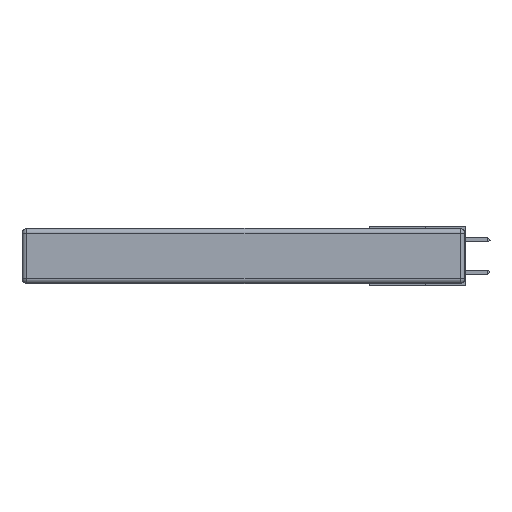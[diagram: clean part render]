
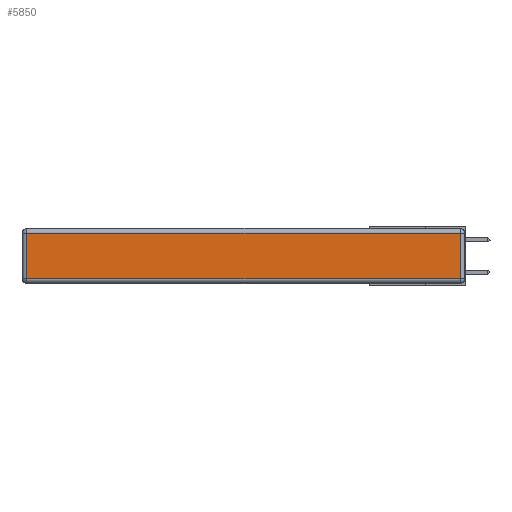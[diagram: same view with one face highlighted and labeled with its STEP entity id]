
A CAD part, left-side view. The second image highlights one B-rep face of the part: STEP entity #5850.
In plain terms, the highlighted planar face has unit normal (-1, 0, 0).
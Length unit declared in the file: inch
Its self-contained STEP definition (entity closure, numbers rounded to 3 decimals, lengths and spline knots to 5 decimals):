
#553 = DIRECTION ( 'NONE',  ( 0., -1., 0. ) ) ;
#827 = CARTESIAN_POINT ( 'NONE',  ( 0., 2.72, -0.343 ) ) ;
#952 = CARTESIAN_POINT ( 'NONE',  ( 0., 0., -0.343 ) ) ;
#1538 = FACE_OUTER_BOUND ( 'NONE', #19409, .T. ) ;
#2417 = CARTESIAN_POINT ( 'NONE',  ( 0., 0., -0.313 ) ) ;
#3534 = CARTESIAN_POINT ( 'NONE',  ( 0., 2.72, -0.03 ) ) ;
#4017 = EDGE_CURVE ( 'NONE', #15215, #13757, #13366, .T. ) ;
#4035 = DIRECTION ( 'NONE',  ( -1., 0., 0. ) ) ;
#4072 = CARTESIAN_POINT ( 'NONE',  ( 0., 0.03, -0.313 ) ) ;
#4230 = EDGE_CURVE ( 'NONE', #11689, #15215, #10212, .T. ) ;
#4703 = VECTOR ( 'NONE', #6827, 39.37008 ) ;
#4950 = CARTESIAN_POINT ( 'NONE',  ( 0., 0.03, -0.03 ) ) ;
#5850 = ADVANCED_FACE ( 'NONE', ( #1538 ), #19548, .T. ) ;
#6288 = CARTESIAN_POINT ( 'NONE',  ( 0., 2.72, -0.313 ) ) ;
#6412 = ORIENTED_EDGE ( 'NONE', *, *, #8215, .T. ) ;
#6415 = ORIENTED_EDGE ( 'NONE', *, *, #4017, .T. ) ;
#6827 = DIRECTION ( 'NONE',  ( 0., 0., -1. ) ) ;
#7492 = CARTESIAN_POINT ( 'NONE',  ( 0., 0.03, -0.343 ) ) ;
#8215 = EDGE_CURVE ( 'NONE', #14708, #11689, #16778, .T. ) ;
#8665 = LINE ( 'NONE', #7492, #10590 ) ;
#9442 = CARTESIAN_POINT ( 'NONE',  ( 0., 2.75, -0.03 ) ) ;
#10212 = LINE ( 'NONE', #827, #4703 ) ;
#10590 = VECTOR ( 'NONE', #19703, 39.37008 ) ;
#10840 = DIRECTION ( 'NONE',  ( 0., 1., 0. ) ) ;
#11382 = ORIENTED_EDGE ( 'NONE', *, *, #4230, .T. ) ;
#11490 = VECTOR ( 'NONE', #10840, 39.37008 ) ;
#11689 = VERTEX_POINT ( 'NONE', #3534 ) ;
#13284 = ORIENTED_EDGE ( 'NONE', *, *, #13407, .T. ) ;
#13366 = LINE ( 'NONE', #2417, #16737 ) ;
#13407 = EDGE_CURVE ( 'NONE', #13757, #14708, #8665, .T. ) ;
#13441 = DIRECTION ( 'NONE',  ( 0., 0., 1. ) ) ;
#13757 = VERTEX_POINT ( 'NONE', #4072 ) ;
#14708 = VERTEX_POINT ( 'NONE', #4950 ) ;
#15215 = VERTEX_POINT ( 'NONE', #6288 ) ;
#16737 = VECTOR ( 'NONE', #553, 39.37008 ) ;
#16778 = LINE ( 'NONE', #9442, #11490 ) ;
#19409 = EDGE_LOOP ( 'NONE', ( #6415, #13284, #6412, #11382 ) ) ;
#19538 = AXIS2_PLACEMENT_3D ( 'NONE', #952, #4035, #13441 ) ;
#19548 = PLANE ( 'NONE',  #19538 ) ;
#19703 = DIRECTION ( 'NONE',  ( 0., 0., 1. ) ) ;
